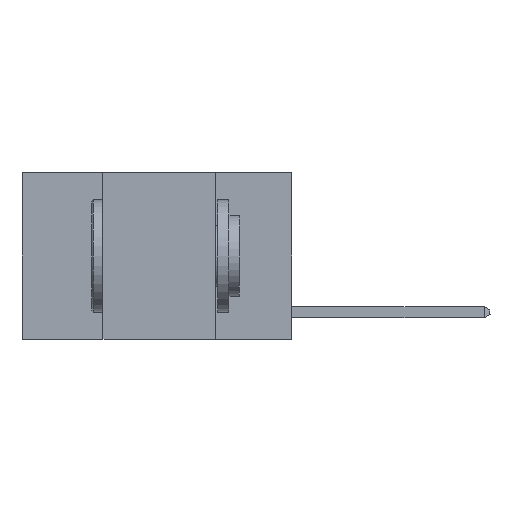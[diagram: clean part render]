
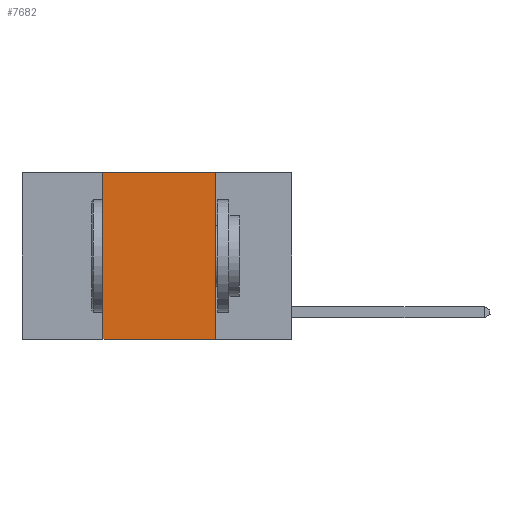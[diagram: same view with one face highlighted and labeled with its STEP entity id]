
A CAD part, left-side view. The second image highlights one B-rep face of the part: STEP entity #7682.
In plain terms, the highlighted planar face has unit normal (-1, 0, 0).
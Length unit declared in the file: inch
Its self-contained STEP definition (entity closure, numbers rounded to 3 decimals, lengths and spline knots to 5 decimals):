
#395 = CARTESIAN_POINT ( 'NONE',  ( 0., 0.6, 0. ) ) ;
#702 = DIRECTION ( 'NONE',  ( 0., -1., 0. ) ) ;
#1106 = VERTEX_POINT ( 'NONE', #5234 ) ;
#1932 = VECTOR ( 'NONE', #9669, 39.37008 ) ;
#2033 = VERTEX_POINT ( 'NONE', #3499 ) ;
#2229 = VERTEX_POINT ( 'NONE', #5543 ) ;
#2347 = DIRECTION ( 'NONE',  ( 0., 0., -1. ) ) ;
#2523 = EDGE_CURVE ( 'NONE', #1106, #2229, #8375, .T. ) ;
#2526 = FACE_OUTER_BOUND ( 'NONE', #3984, .T. ) ;
#2712 = EDGE_CURVE ( 'NONE', #2229, #5151, #4944, .T. ) ;
#2763 = VECTOR ( 'NONE', #702, 39.37008 ) ;
#3266 = EDGE_CURVE ( 'NONE', #2033, #1106, #8734, .T. ) ;
#3499 = CARTESIAN_POINT ( 'NONE',  ( 0., 0.42, -0.37 ) ) ;
#3785 = EDGE_CURVE ( 'NONE', #2033, #5151, #4323, .T. ) ;
#3984 = EDGE_LOOP ( 'NONE', ( #5949, #7863, #6042, #10089 ) ) ;
#4323 = LINE ( 'NONE', #6497, #1932 ) ;
#4483 = DIRECTION ( 'NONE',  ( 0., 0., -1. ) ) ;
#4672 = AXIS2_PLACEMENT_3D ( 'NONE', #395, #6518, #4483 ) ;
#4940 = DIRECTION ( 'NONE',  ( 0., 0., 1. ) ) ;
#4944 = LINE ( 'NONE', #8021, #5405 ) ;
#5151 = VERTEX_POINT ( 'NONE', #5259 ) ;
#5234 = CARTESIAN_POINT ( 'NONE',  ( 0., 0.42, 0. ) ) ;
#5259 = CARTESIAN_POINT ( 'NONE',  ( 0., 0.17, -0.37 ) ) ;
#5405 = VECTOR ( 'NONE', #2347, 39.37008 ) ;
#5543 = CARTESIAN_POINT ( 'NONE',  ( 0., 0.17, 0. ) ) ;
#5949 = ORIENTED_EDGE ( 'NONE', *, *, #2712, .F. ) ;
#6042 = ORIENTED_EDGE ( 'NONE', *, *, #3266, .F. ) ;
#6497 = CARTESIAN_POINT ( 'NONE',  ( 0., 0.6, -0.37 ) ) ;
#6518 = DIRECTION ( 'NONE',  ( 1., 0., 0. ) ) ;
#7682 = ADVANCED_FACE ( 'NONE', ( #2526 ), #9100, .F. ) ;
#7807 = CARTESIAN_POINT ( 'NONE',  ( 0., 0.6, 0. ) ) ;
#7863 = ORIENTED_EDGE ( 'NONE', *, *, #2523, .F. ) ;
#8021 = CARTESIAN_POINT ( 'NONE',  ( 0., 0.17, 0. ) ) ;
#8375 = LINE ( 'NONE', #7807, #2763 ) ;
#8734 = LINE ( 'NONE', #8893, #8744 ) ;
#8744 = VECTOR ( 'NONE', #4940, 39.37008 ) ;
#8893 = CARTESIAN_POINT ( 'NONE',  ( 0., 0.42, 0. ) ) ;
#9100 = PLANE ( 'NONE',  #4672 ) ;
#9669 = DIRECTION ( 'NONE',  ( 0., -1., 0. ) ) ;
#10089 = ORIENTED_EDGE ( 'NONE', *, *, #3785, .T. ) ;
